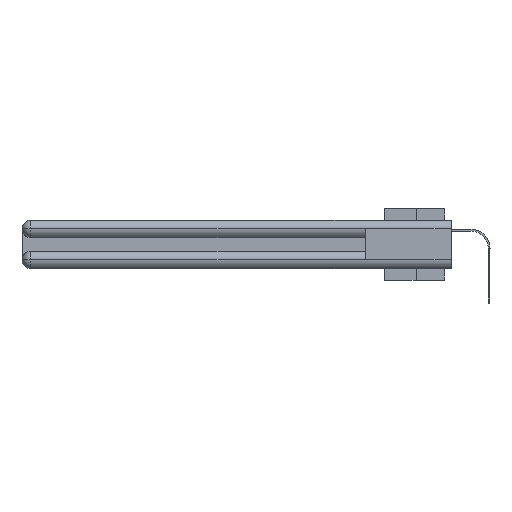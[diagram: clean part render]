
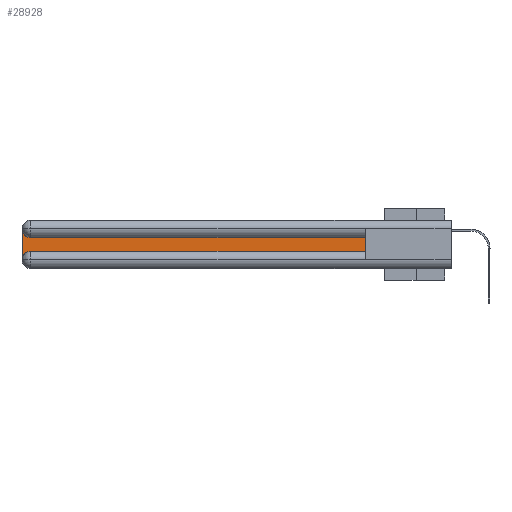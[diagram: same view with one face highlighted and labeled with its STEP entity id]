
A CAD part, left-side view. The second image highlights one B-rep face of the part: STEP entity #28928.
In plain terms, the highlighted planar face has unit normal (-1, 0, 0).
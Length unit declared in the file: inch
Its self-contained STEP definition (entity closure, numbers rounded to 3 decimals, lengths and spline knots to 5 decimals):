
#990 = DIRECTION ( 'NONE',  ( 1., 0., 0. ) ) ;
#1074 = AXIS2_PLACEMENT_3D ( 'NONE', #33113, #990, #27143 ) ;
#1084 = AXIS2_PLACEMENT_3D ( 'NONE', #24559, #3789, #1671 ) ;
#1671 = DIRECTION ( 'NONE',  ( 0., 0., -1. ) ) ;
#3789 = DIRECTION ( 'NONE',  ( 1., 0., 0. ) ) ;
#3916 = EDGE_CURVE ( 'NONE', #8573, #8544, #14627, .T. ) ;
#4026 = CARTESIAN_POINT ( 'NONE',  ( 0.075, 0.6, -0.1225 ) ) ;
#5638 = DIRECTION ( 'NONE',  ( 0., 0., -1. ) ) ;
#6468 = ORIENTED_EDGE ( 'NONE', *, *, #14211, .T. ) ;
#7469 = VERTEX_POINT ( 'NONE', #32674 ) ;
#7727 = DIRECTION ( 'NONE',  ( 0., 0., -1. ) ) ;
#8544 = VERTEX_POINT ( 'NONE', #19512 ) ;
#8573 = VERTEX_POINT ( 'NONE', #25471 ) ;
#8968 = ORIENTED_EDGE ( 'NONE', *, *, #3916, .T. ) ;
#11002 = VERTEX_POINT ( 'NONE', #12470 ) ;
#11390 = CARTESIAN_POINT ( 'NONE',  ( 0.075, 0.6, -0.2175 ) ) ;
#11497 = CIRCLE ( 'NONE', #21934, 0.06 ) ;
#11789 = CARTESIAN_POINT ( 'NONE',  ( 0.075, 3., -0.2175 ) ) ;
#11881 = VECTOR ( 'NONE', #5638, 39.37008 ) ;
#12470 = CARTESIAN_POINT ( 'NONE',  ( 0.075, 0.6, -0.1225 ) ) ;
#14211 = EDGE_CURVE ( 'NONE', #7469, #11002, #29058, .T. ) ;
#14465 = VERTEX_POINT ( 'NONE', #21909 ) ;
#14627 = CIRCLE ( 'NONE', #1074, 0.06 ) ;
#16296 = LINE ( 'NONE', #25132, #21306 ) ;
#16336 = DIRECTION ( 'NONE',  ( 0., 1., 0. ) ) ;
#16682 = ORIENTED_EDGE ( 'NONE', *, *, #28108, .T. ) ;
#19117 = EDGE_CURVE ( 'NONE', #8544, #33693, #26766, .T. ) ;
#19512 = CARTESIAN_POINT ( 'NONE',  ( 0.075, 3., -0.0625 ) ) ;
#20125 = EDGE_CURVE ( 'NONE', #11002, #8573, #25367, .T. ) ;
#21306 = VECTOR ( 'NONE', #22066, 39.37008 ) ;
#21909 = CARTESIAN_POINT ( 'NONE',  ( 0.075, 2.94, -0.2175 ) ) ;
#21934 = AXIS2_PLACEMENT_3D ( 'NONE', #24654, #25038, #7727 ) ;
#22066 = DIRECTION ( 'NONE',  ( 0., -1., 0. ) ) ;
#22533 = DIRECTION ( 'NONE',  ( 0., 0., 1. ) ) ;
#24366 = FACE_OUTER_BOUND ( 'NONE', #26301, .T. ) ;
#24559 = CARTESIAN_POINT ( 'NONE',  ( 0.075, 3., -0.1225 ) ) ;
#24654 = CARTESIAN_POINT ( 'NONE',  ( 0.075, 2.94, -0.2775 ) ) ;
#25038 = DIRECTION ( 'NONE',  ( 1., 0., 0. ) ) ;
#25132 = CARTESIAN_POINT ( 'NONE',  ( 0.075, 0.6, -0.2175 ) ) ;
#25367 = LINE ( 'NONE', #4026, #32218 ) ;
#25471 = CARTESIAN_POINT ( 'NONE',  ( 0.075, 2.94, -0.1225 ) ) ;
#25727 = EDGE_CURVE ( 'NONE', #14465, #7469, #16296, .T. ) ;
#26301 = EDGE_LOOP ( 'NONE', ( #36860, #8968, #36711, #16682, #27287, #6468 ) ) ;
#26766 = LINE ( 'NONE', #11789, #11881 ) ;
#27143 = DIRECTION ( 'NONE',  ( 0., 0., -1. ) ) ;
#27287 = ORIENTED_EDGE ( 'NONE', *, *, #25727, .T. ) ;
#27451 = PLANE ( 'NONE',  #1084 ) ;
#28108 = EDGE_CURVE ( 'NONE', #33693, #14465, #11497, .T. ) ;
#28928 = ADVANCED_FACE ( 'NONE', ( #24366 ), #27451, .F. ) ;
#29058 = LINE ( 'NONE', #11390, #29341 ) ;
#29341 = VECTOR ( 'NONE', #22533, 39.37008 ) ;
#32218 = VECTOR ( 'NONE', #16336, 39.37008 ) ;
#32674 = CARTESIAN_POINT ( 'NONE',  ( 0.075, 0.6, -0.2175 ) ) ;
#33113 = CARTESIAN_POINT ( 'NONE',  ( 0.075, 2.94, -0.0625 ) ) ;
#33693 = VERTEX_POINT ( 'NONE', #36352 ) ;
#36352 = CARTESIAN_POINT ( 'NONE',  ( 0.075, 3., -0.2775 ) ) ;
#36711 = ORIENTED_EDGE ( 'NONE', *, *, #19117, .T. ) ;
#36860 = ORIENTED_EDGE ( 'NONE', *, *, #20125, .T. ) ;
